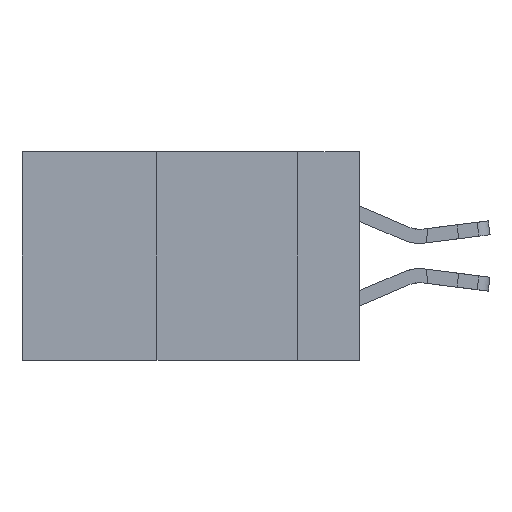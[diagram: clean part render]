
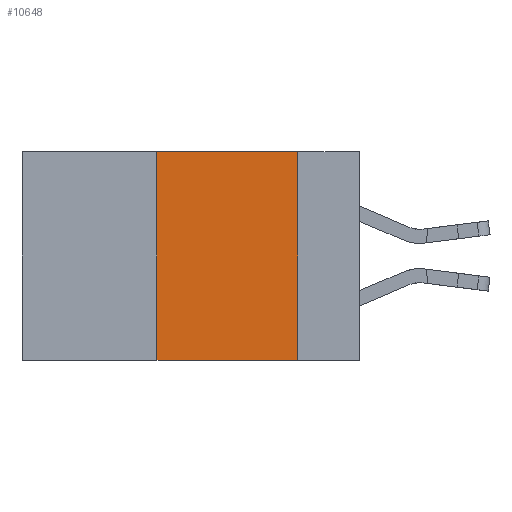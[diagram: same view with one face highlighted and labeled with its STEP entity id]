
A CAD part, left-side view. The second image highlights one B-rep face of the part: STEP entity #10648.
In plain terms, the highlighted planar face has unit normal (-1, 0, 0).
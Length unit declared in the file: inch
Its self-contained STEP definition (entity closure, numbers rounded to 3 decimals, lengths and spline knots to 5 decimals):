
#257 = CARTESIAN_POINT ( 'NONE',  ( 0., 0.6, 0. ) ) ;
#801 = DIRECTION ( 'NONE',  ( 0., 0., -1. ) ) ;
#954 = CARTESIAN_POINT ( 'NONE',  ( 0., 0.11, -0.37 ) ) ;
#1183 = PLANE ( 'NONE',  #7337 ) ;
#1631 = VERTEX_POINT ( 'NONE', #3635 ) ;
#2672 = EDGE_CURVE ( 'NONE', #11933, #14920, #7843, .T. ) ;
#3189 = ORIENTED_EDGE ( 'NONE', *, *, #9062, .F. ) ;
#3635 = CARTESIAN_POINT ( 'NONE',  ( 0., 0.36, -0.37 ) ) ;
#4233 = DIRECTION ( 'NONE',  ( 1., 0., 0. ) ) ;
#4442 = LINE ( 'NONE', #257, #9087 ) ;
#5114 = DIRECTION ( 'NONE',  ( 0., -1., 0. ) ) ;
#6158 = ORIENTED_EDGE ( 'NONE', *, *, #2672, .F. ) ;
#7055 = VECTOR ( 'NONE', #801, 39.37008 ) ;
#7300 = VECTOR ( 'NONE', #5114, 39.37008 ) ;
#7337 = AXIS2_PLACEMENT_3D ( 'NONE', #8850, #4233, #8580 ) ;
#7843 = LINE ( 'NONE', #10972, #7055 ) ;
#8153 = CARTESIAN_POINT ( 'NONE',  ( 0., 0.6, -0.37 ) ) ;
#8580 = DIRECTION ( 'NONE',  ( 0., 0., -1. ) ) ;
#8850 = CARTESIAN_POINT ( 'NONE',  ( 0., 0.6, 0. ) ) ;
#9062 = EDGE_CURVE ( 'NONE', #9458, #11933, #4442, .T. ) ;
#9087 = VECTOR ( 'NONE', #11626, 39.37008 ) ;
#9458 = VERTEX_POINT ( 'NONE', #11422 ) ;
#10648 = ADVANCED_FACE ( 'NONE', ( #10980 ), #1183, .F. ) ;
#10972 = CARTESIAN_POINT ( 'NONE',  ( 0., 0.11, 0. ) ) ;
#10980 = FACE_OUTER_BOUND ( 'NONE', #14725, .T. ) ;
#11146 = ORIENTED_EDGE ( 'NONE', *, *, #17376, .F. ) ;
#11422 = CARTESIAN_POINT ( 'NONE',  ( 0., 0.36, 0. ) ) ;
#11626 = DIRECTION ( 'NONE',  ( 0., -1., 0. ) ) ;
#11933 = VERTEX_POINT ( 'NONE', #12636 ) ;
#12636 = CARTESIAN_POINT ( 'NONE',  ( 0., 0.11, 0. ) ) ;
#13587 = ORIENTED_EDGE ( 'NONE', *, *, #14929, .T. ) ;
#14725 = EDGE_LOOP ( 'NONE', ( #6158, #3189, #11146, #13587 ) ) ;
#14920 = VERTEX_POINT ( 'NONE', #954 ) ;
#14929 = EDGE_CURVE ( 'NONE', #1631, #14920, #17848, .T. ) ;
#14962 = CARTESIAN_POINT ( 'NONE',  ( 0., 0.36, 0. ) ) ;
#15864 = VECTOR ( 'NONE', #18010, 39.37008 ) ;
#16455 = LINE ( 'NONE', #14962, #15864 ) ;
#17376 = EDGE_CURVE ( 'NONE', #1631, #9458, #16455, .T. ) ;
#17848 = LINE ( 'NONE', #8153, #7300 ) ;
#18010 = DIRECTION ( 'NONE',  ( 0., 0., 1. ) ) ;
